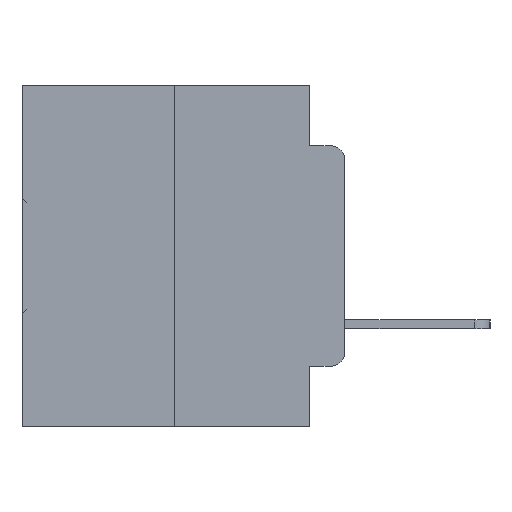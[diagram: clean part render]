
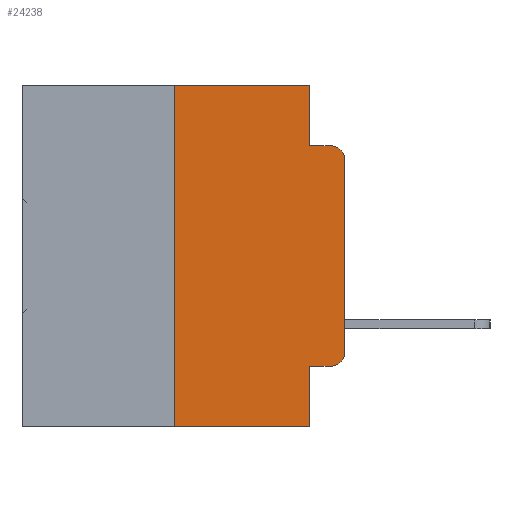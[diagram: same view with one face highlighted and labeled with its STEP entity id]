
A CAD part, left-side view. The second image highlights one B-rep face of the part: STEP entity #24238.
In plain terms, the highlighted planar face has unit normal (-1, 0, 0).
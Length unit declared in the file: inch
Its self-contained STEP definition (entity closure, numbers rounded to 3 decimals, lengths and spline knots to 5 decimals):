
#327 = EDGE_CURVE ( 'NONE', #20010, #27016, #15634, .T. ) ;
#602 = CARTESIAN_POINT ( 'NONE',  ( 0., 0., -0.3915 ) ) ;
#902 = CARTESIAN_POINT ( 'NONE',  ( 0., 0.25, 0. ) ) ;
#949 = DIRECTION ( 'NONE',  ( 0., 0., -1. ) ) ;
#2127 = EDGE_LOOP ( 'NONE', ( #14865, #2237, #8986, #16466, #18820, #26813, #14491, #21904, #9397, #22663 ) ) ;
#2237 = ORIENTED_EDGE ( 'NONE', *, *, #20602, .T. ) ;
#3004 = DIRECTION ( 'NONE',  ( 0., -1., 0. ) ) ;
#3128 = VECTOR ( 'NONE', #10085, 39.37008 ) ;
#3998 = CARTESIAN_POINT ( 'NONE',  ( 0., 0.473, 0. ) ) ;
#4230 = CARTESIAN_POINT ( 'NONE',  ( 0., 0.02, -0.3915 ) ) ;
#4623 = EDGE_CURVE ( 'NONE', #20010, #12902, #30662, .T. ) ;
#4838 = LINE ( 'NONE', #13547, #15062 ) ;
#5005 = CARTESIAN_POINT ( 'NONE',  ( 0., 0., 0. ) ) ;
#5459 = EDGE_CURVE ( 'NONE', #15637, #21334, #20897, .T. ) ;
#5652 = LINE ( 'NONE', #24435, #18247 ) ;
#5883 = VERTEX_POINT ( 'NONE', #6011 ) ;
#6011 = CARTESIAN_POINT ( 'NONE',  ( 0., 0.02, -0.4115 ) ) ;
#6090 = EDGE_CURVE ( 'NONE', #5883, #26392, #10295, .T. ) ;
#6546 = DIRECTION ( 'NONE',  ( 0., 0., -1. ) ) ;
#6781 = DIRECTION ( 'NONE',  ( 0., 0., -1. ) ) ;
#8986 = ORIENTED_EDGE ( 'NONE', *, *, #13895, .F. ) ;
#9397 = ORIENTED_EDGE ( 'NONE', *, *, #19554, .T. ) ;
#9545 = DIRECTION ( 'NONE',  ( 0., -1., 0. ) ) ;
#9729 = VECTOR ( 'NONE', #22984, 39.37008 ) ;
#9824 = CARTESIAN_POINT ( 'NONE',  ( 0., 0.051, -0.0885 ) ) ;
#10085 = DIRECTION ( 'NONE',  ( 0., 0., 1. ) ) ;
#10230 = DIRECTION ( 'NONE',  ( -1., 0., 0. ) ) ;
#10295 = CIRCLE ( 'NONE', #20469, 0.02 ) ;
#10615 = CARTESIAN_POINT ( 'NONE',  ( 0., 0.473, -0.5 ) ) ;
#11658 = LINE ( 'NONE', #9824, #17525 ) ;
#12179 = CARTESIAN_POINT ( 'NONE',  ( 0., 0.051, -0.4115 ) ) ;
#12280 = CARTESIAN_POINT ( 'NONE',  ( 0., 0.25, 0. ) ) ;
#12902 = VERTEX_POINT ( 'NONE', #25518 ) ;
#13075 = AXIS2_PLACEMENT_3D ( 'NONE', #3998, #21528, #6546 ) ;
#13547 = CARTESIAN_POINT ( 'NONE',  ( 0., 0.051, 0. ) ) ;
#13895 = EDGE_CURVE ( 'NONE', #21334, #23110, #11658, .T. ) ;
#14007 = PLANE ( 'NONE',  #13075 ) ;
#14311 = CARTESIAN_POINT ( 'NONE',  ( 0., 0.051, 0. ) ) ;
#14491 = ORIENTED_EDGE ( 'NONE', *, *, #4623, .T. ) ;
#14856 = DIRECTION ( 'NONE',  ( 0., -1., 0. ) ) ;
#14865 = ORIENTED_EDGE ( 'NONE', *, *, #23871, .T. ) ;
#15029 = VECTOR ( 'NONE', #16485, 39.37008 ) ;
#15060 = LINE ( 'NONE', #27738, #20154 ) ;
#15062 = VECTOR ( 'NONE', #949, 39.37008 ) ;
#15634 = LINE ( 'NONE', #12280, #9729 ) ;
#15637 = VERTEX_POINT ( 'NONE', #14311 ) ;
#16466 = ORIENTED_EDGE ( 'NONE', *, *, #5459, .F. ) ;
#16479 = CARTESIAN_POINT ( 'NONE',  ( 0., 0., -0.1085 ) ) ;
#16485 = DIRECTION ( 'NONE',  ( 0., 0., -1. ) ) ;
#16523 = LINE ( 'NONE', #5005, #3128 ) ;
#17525 = VECTOR ( 'NONE', #14856, 39.37008 ) ;
#17854 = VECTOR ( 'NONE', #27720, 39.37008 ) ;
#18247 = VECTOR ( 'NONE', #9545, 39.37008 ) ;
#18820 = ORIENTED_EDGE ( 'NONE', *, *, #21045, .F. ) ;
#19554 = EDGE_CURVE ( 'NONE', #23762, #5883, #15060, .T. ) ;
#20010 = VERTEX_POINT ( 'NONE', #31849 ) ;
#20154 = VECTOR ( 'NONE', #3004, 39.37008 ) ;
#20469 = AXIS2_PLACEMENT_3D ( 'NONE', #4230, #21763, #6781 ) ;
#20602 = EDGE_CURVE ( 'NONE', #23567, #23110, #24786, .T. ) ;
#20897 = LINE ( 'NONE', #28596, #15029 ) ;
#21045 = EDGE_CURVE ( 'NONE', #27016, #15637, #5652, .T. ) ;
#21334 = VERTEX_POINT ( 'NONE', #23027 ) ;
#21528 = DIRECTION ( 'NONE',  ( 1., 0., 0. ) ) ;
#21763 = DIRECTION ( 'NONE',  ( -1., 0., 0. ) ) ;
#21904 = ORIENTED_EDGE ( 'NONE', *, *, #29210, .F. ) ;
#22663 = ORIENTED_EDGE ( 'NONE', *, *, #6090, .T. ) ;
#22984 = DIRECTION ( 'NONE',  ( 0., 0., 1. ) ) ;
#23027 = CARTESIAN_POINT ( 'NONE',  ( 0., 0.051, -0.0885 ) ) ;
#23110 = VERTEX_POINT ( 'NONE', #28906 ) ;
#23567 = VERTEX_POINT ( 'NONE', #16479 ) ;
#23762 = VERTEX_POINT ( 'NONE', #12179 ) ;
#23831 = AXIS2_PLACEMENT_3D ( 'NONE', #25099, #10230, #27475 ) ;
#23871 = EDGE_CURVE ( 'NONE', #26392, #23567, #16523, .T. ) ;
#24238 = ADVANCED_FACE ( 'NONE', ( #29357 ), #14007, .F. ) ;
#24435 = CARTESIAN_POINT ( 'NONE',  ( 0., 0.473, 0. ) ) ;
#24786 = CIRCLE ( 'NONE', #23831, 0.02 ) ;
#25099 = CARTESIAN_POINT ( 'NONE',  ( 0., 0.02, -0.1085 ) ) ;
#25518 = CARTESIAN_POINT ( 'NONE',  ( 0., 0.051, -0.5 ) ) ;
#26392 = VERTEX_POINT ( 'NONE', #602 ) ;
#26813 = ORIENTED_EDGE ( 'NONE', *, *, #327, .F. ) ;
#27016 = VERTEX_POINT ( 'NONE', #902 ) ;
#27475 = DIRECTION ( 'NONE',  ( 0., 0., -1. ) ) ;
#27720 = DIRECTION ( 'NONE',  ( 0., -1., 0. ) ) ;
#27738 = CARTESIAN_POINT ( 'NONE',  ( 0., 0.051, -0.4115 ) ) ;
#28596 = CARTESIAN_POINT ( 'NONE',  ( 0., 0.051, 0. ) ) ;
#28906 = CARTESIAN_POINT ( 'NONE',  ( 0., 0.02, -0.0885 ) ) ;
#29210 = EDGE_CURVE ( 'NONE', #23762, #12902, #4838, .T. ) ;
#29357 = FACE_OUTER_BOUND ( 'NONE', #2127, .T. ) ;
#30662 = LINE ( 'NONE', #10615, #17854 ) ;
#31849 = CARTESIAN_POINT ( 'NONE',  ( 0., 0.25, -0.5 ) ) ;
